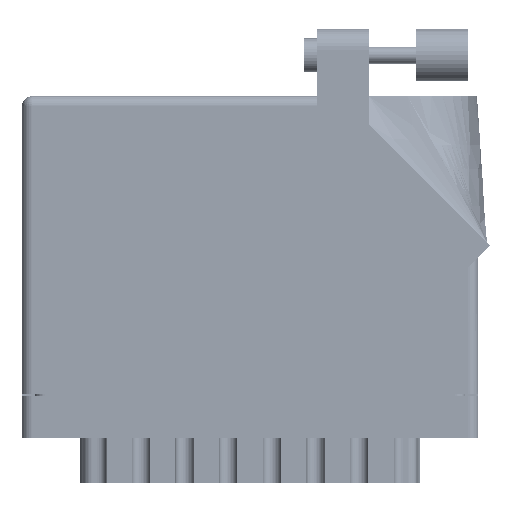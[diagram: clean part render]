
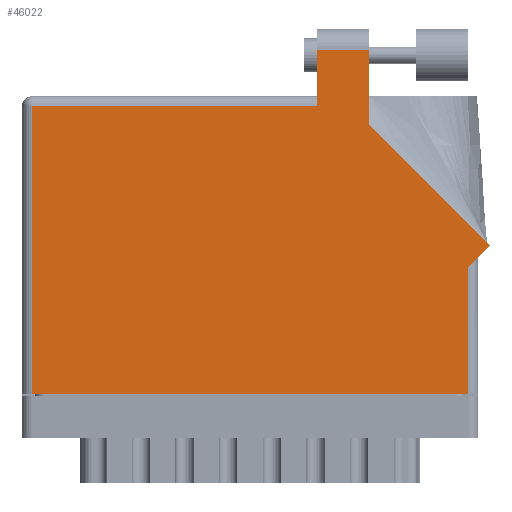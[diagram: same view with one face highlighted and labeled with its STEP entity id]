
A CAD part, front view. The second image highlights one B-rep face of the part: STEP entity #46022.
In plain terms, the highlighted face is planar.
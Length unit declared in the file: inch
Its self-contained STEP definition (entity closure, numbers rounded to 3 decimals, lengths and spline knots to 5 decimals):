
#1546 = VERTEX_POINT ( 'NONE', #16436 ) ;
#1773 = LINE ( 'NONE', #41803, #72898 ) ;
#2423 = EDGE_CURVE ( 'NONE', #70973, #35022, #24184, .T. ) ;
#3685 = VECTOR ( 'NONE', #35772, 39.37008 ) ;
#3797 = VERTEX_POINT ( 'NONE', #22652 ) ;
#5498 = VECTOR ( 'NONE', #34608, 39.37008 ) ;
#7048 = VERTEX_POINT ( 'NONE', #64345 ) ;
#7142 = VERTEX_POINT ( 'NONE', #47783 ) ;
#8324 = LINE ( 'NONE', #15728, #12103 ) ;
#9578 = EDGE_CURVE ( 'NONE', #7142, #69558, #11780, .T. ) ;
#11780 = LINE ( 'NONE', #51759, #53302 ) ;
#12103 = VECTOR ( 'NONE', #22419, 39.37008 ) ;
#12276 = CARTESIAN_POINT ( 'NONE',  ( 2.78871, 0.88571, 0. ) ) ;
#15327 = ORIENTED_EDGE ( 'NONE', *, *, #75891, .T. ) ;
#15728 = CARTESIAN_POINT ( 'NONE',  ( 2.656, 0.815, 0. ) ) ;
#16378 = CARTESIAN_POINT ( 'NONE',  ( 0., 1.775, 0. ) ) ;
#16436 = CARTESIAN_POINT ( 'NONE',  ( 2.065, 1.60942, 0. ) ) ;
#16596 = VERTEX_POINT ( 'NONE', #29659 ) ;
#19268 = ORIENTED_EDGE ( 'NONE', *, *, #54247, .T. ) ;
#19577 = CARTESIAN_POINT ( 'NONE',  ( 1.758, 1.775, 0. ) ) ;
#21228 = LINE ( 'NONE', #28929, #5498 ) ;
#21584 = LINE ( 'NONE', #64859, #60371 ) ;
#22019 = LINE ( 'NONE', #29088, #3685 ) ;
#22419 = DIRECTION ( 'NONE',  ( 0., 1., 0. ) ) ;
#22652 = CARTESIAN_POINT ( 'NONE',  ( 2.656, 0., 0. ) ) ;
#22882 = DIRECTION ( 'NONE',  ( -1., 0., 0. ) ) ;
#24184 = LINE ( 'NONE', #19577, #45439 ) ;
#25480 = EDGE_CURVE ( 'NONE', #16596, #7048, #31861, .T. ) ;
#28322 = DIRECTION ( 'NONE',  ( 0.707, 0.707, 0. ) ) ;
#28825 = CARTESIAN_POINT ( 'NONE',  ( 0.062, 0., 0. ) ) ;
#28929 = CARTESIAN_POINT ( 'NONE',  ( 2.065, 1.60942, 0. ) ) ;
#29088 = CARTESIAN_POINT ( 'NONE',  ( 2.78871, 0.88571, 0. ) ) ;
#29659 = CARTESIAN_POINT ( 'NONE',  ( 0.062, 1.713, 0. ) ) ;
#30543 = EDGE_LOOP ( 'NONE', ( #54641, #19268, #50163, #41629, #48730, #15327, #58295, #69591, #34108 ) ) ;
#31861 = LINE ( 'NONE', #28825, #33695 ) ;
#32798 = EDGE_CURVE ( 'NONE', #1546, #70121, #21228, .T. ) ;
#33461 = EDGE_CURVE ( 'NONE', #69558, #1546, #22019, .T. ) ;
#33695 = VECTOR ( 'NONE', #69876, 39.37008 ) ;
#34108 = ORIENTED_EDGE ( 'NONE', *, *, #33461, .T. ) ;
#34151 = CARTESIAN_POINT ( 'NONE',  ( 1.758, 2.05, 0. ) ) ;
#34608 = DIRECTION ( 'NONE',  ( 0., 1., 0. ) ) ;
#35022 = VERTEX_POINT ( 'NONE', #65965 ) ;
#35772 = DIRECTION ( 'NONE',  ( -0.707, 0.707, 0. ) ) ;
#37126 = DIRECTION ( 'NONE',  ( 0., -1., 0. ) ) ;
#41629 = ORIENTED_EDGE ( 'NONE', *, *, #58840, .T. ) ;
#41803 = CARTESIAN_POINT ( 'NONE',  ( 0., 0., 0. ) ) ;
#45439 = VECTOR ( 'NONE', #37126, 39.37008 ) ;
#45460 = FACE_OUTER_BOUND ( 'NONE', #30543, .T. ) ;
#45685 = VECTOR ( 'NONE', #22882, 39.37008 ) ;
#46022 = ADVANCED_FACE ( 'NONE', ( #45460 ), #51691, .F. ) ;
#47060 = EDGE_CURVE ( 'NONE', #3797, #7142, #8324, .T. ) ;
#47284 = DIRECTION ( 'NONE',  ( -1., 0., 0. ) ) ;
#47783 = CARTESIAN_POINT ( 'NONE',  ( 2.656, 0.753, 0. ) ) ;
#48730 = ORIENTED_EDGE ( 'NONE', *, *, #25480, .T. ) ;
#50163 = ORIENTED_EDGE ( 'NONE', *, *, #2423, .T. ) ;
#51262 = CARTESIAN_POINT ( 'NONE',  ( 1.758, 2.05, 0. ) ) ;
#51691 = PLANE ( 'NONE',  #68210 ) ;
#51759 = CARTESIAN_POINT ( 'NONE',  ( 2.718, 0.815, 0. ) ) ;
#53302 = VECTOR ( 'NONE', #28322, 39.37008 ) ;
#53329 = DIRECTION ( 'NONE',  ( 1., 0., 0. ) ) ;
#54247 = EDGE_CURVE ( 'NONE', #70121, #70973, #58589, .T. ) ;
#54641 = ORIENTED_EDGE ( 'NONE', *, *, #32798, .T. ) ;
#58295 = ORIENTED_EDGE ( 'NONE', *, *, #47060, .T. ) ;
#58589 = LINE ( 'NONE', #51262, #45685 ) ;
#58650 = DIRECTION ( 'NONE',  ( -1., 0., 0. ) ) ;
#58840 = EDGE_CURVE ( 'NONE', #35022, #16596, #21584, .T. ) ;
#60371 = VECTOR ( 'NONE', #47284, 39.37008 ) ;
#64345 = CARTESIAN_POINT ( 'NONE',  ( 0.062, 0., 0. ) ) ;
#64859 = CARTESIAN_POINT ( 'NONE',  ( 0., 1.713, 0. ) ) ;
#65965 = CARTESIAN_POINT ( 'NONE',  ( 1.758, 1.713, 0. ) ) ;
#68210 = AXIS2_PLACEMENT_3D ( 'NONE', #16378, #76036, #58650 ) ;
#69558 = VERTEX_POINT ( 'NONE', #12276 ) ;
#69591 = ORIENTED_EDGE ( 'NONE', *, *, #9578, .T. ) ;
#69876 = DIRECTION ( 'NONE',  ( 0., -1., 0. ) ) ;
#70121 = VERTEX_POINT ( 'NONE', #73579 ) ;
#70973 = VERTEX_POINT ( 'NONE', #34151 ) ;
#72898 = VECTOR ( 'NONE', #53329, 39.37008 ) ;
#73579 = CARTESIAN_POINT ( 'NONE',  ( 2.065, 2.05, 0. ) ) ;
#75891 = EDGE_CURVE ( 'NONE', #7048, #3797, #1773, .T. ) ;
#76036 = DIRECTION ( 'NONE',  ( 0., 0., -1. ) ) ;
